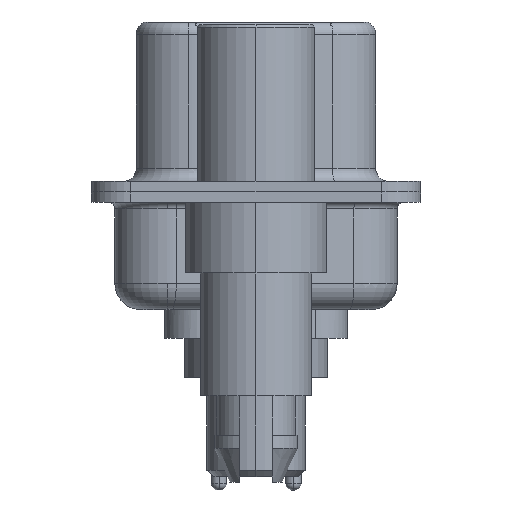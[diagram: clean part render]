
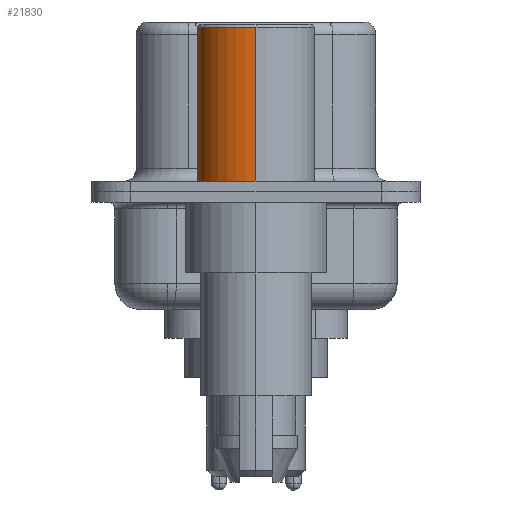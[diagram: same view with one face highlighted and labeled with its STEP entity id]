
A CAD part, left-side view. The second image highlights one B-rep face of the part: STEP entity #21830.
In plain terms, the highlighted cylindrical face has radius 2.25 mm (diameter 4.5 mm), a partial arc.
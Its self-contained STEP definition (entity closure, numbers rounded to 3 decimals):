
#266 = EDGE_LOOP ( 'NONE', ( #21541, #18764, #12326, #9480 ) ) ;
#291 = AXIS2_PLACEMENT_3D ( 'NONE', #19591, #9425, #21242 ) ;
#1224 = EDGE_CURVE ( 'NONE', #5790, #7825, #2334, .T. ) ;
#1783 = CARTESIAN_POINT ( 'NONE',  ( -2.25, 0., 6.3 ) ) ;
#2036 = CIRCLE ( 'NONE', #291, 2.25 ) ;
#2334 = LINE ( 'NONE', #7230, #15304 ) ;
#2507 = FACE_OUTER_BOUND ( 'NONE', #266, .T. ) ;
#3371 = CARTESIAN_POINT ( 'NONE',  ( -2.25, 0., 0.581 ) ) ;
#5790 = VERTEX_POINT ( 'NONE', #17159 ) ;
#6478 = CYLINDRICAL_SURFACE ( 'NONE', #18466, 2.25 ) ;
#7230 = CARTESIAN_POINT ( 'NONE',  ( 2.25, 0., 0.581 ) ) ;
#7825 = VERTEX_POINT ( 'NONE', #20210 ) ;
#8355 = DIRECTION ( 'NONE',  ( 0., 0., 1. ) ) ;
#8675 = DIRECTION ( 'NONE',  ( 0., 0., 1. ) ) ;
#8727 = EDGE_CURVE ( 'NONE', #10052, #20487, #13741, .T. ) ;
#8870 = DIRECTION ( 'NONE',  ( 0., 0., 1. ) ) ;
#8922 = CARTESIAN_POINT ( 'NONE',  ( -2.25, 0., 0.4 ) ) ;
#9044 = AXIS2_PLACEMENT_3D ( 'NONE', #18494, #8355, #20185 ) ;
#9425 = DIRECTION ( 'NONE',  ( 0., 0., 1. ) ) ;
#9480 = ORIENTED_EDGE ( 'NONE', *, *, #1224, .F. ) ;
#10052 = VERTEX_POINT ( 'NONE', #8922 ) ;
#12050 = DIRECTION ( 'NONE',  ( 1., 0., 0. ) ) ;
#12326 = ORIENTED_EDGE ( 'NONE', *, *, #19244, .F. ) ;
#13192 = VECTOR ( 'NONE', #15166, 1000. ) ;
#13741 = LINE ( 'NONE', #3371, #13192 ) ;
#15166 = DIRECTION ( 'NONE',  ( 0., 0., 1. ) ) ;
#15304 = VECTOR ( 'NONE', #8870, 1000. ) ;
#15389 = CARTESIAN_POINT ( 'NONE',  ( 0., 0., 0.581 ) ) ;
#17159 = CARTESIAN_POINT ( 'NONE',  ( 2.25, 0., 0.4 ) ) ;
#17948 = CIRCLE ( 'NONE', #9044, 2.25 ) ;
#18466 = AXIS2_PLACEMENT_3D ( 'NONE', #15389, #8675, #12050 ) ;
#18494 = CARTESIAN_POINT ( 'NONE',  ( 0., 0., 6.3 ) ) ;
#18764 = ORIENTED_EDGE ( 'NONE', *, *, #8727, .T. ) ;
#19244 = EDGE_CURVE ( 'NONE', #7825, #20487, #17948, .T. ) ;
#19591 = CARTESIAN_POINT ( 'NONE',  ( 0., 0., 0.4 ) ) ;
#19659 = EDGE_CURVE ( 'NONE', #5790, #10052, #2036, .T. ) ;
#20185 = DIRECTION ( 'NONE',  ( 1., 0., 0. ) ) ;
#20210 = CARTESIAN_POINT ( 'NONE',  ( 2.25, 0., 6.3 ) ) ;
#20487 = VERTEX_POINT ( 'NONE', #1783 ) ;
#21242 = DIRECTION ( 'NONE',  ( 1., 0., 0. ) ) ;
#21541 = ORIENTED_EDGE ( 'NONE', *, *, #19659, .T. ) ;
#21830 = ADVANCED_FACE ( 'NONE', ( #2507 ), #6478, .T. ) ;
